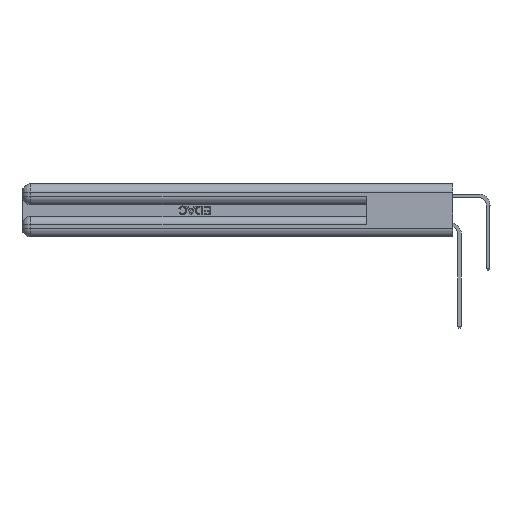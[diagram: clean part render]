
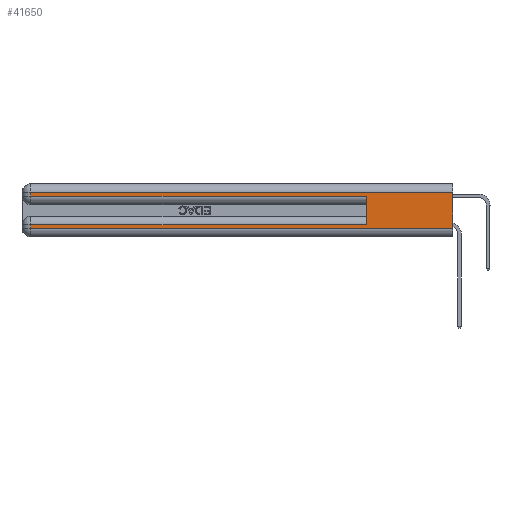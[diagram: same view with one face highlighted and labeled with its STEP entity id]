
A CAD part, left-side view. The second image highlights one B-rep face of the part: STEP entity #41650.
In plain terms, the highlighted planar face has unit normal (-1, 0, 0).
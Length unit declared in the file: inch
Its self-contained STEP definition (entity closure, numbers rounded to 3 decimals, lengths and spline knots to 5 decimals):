
#1185 = CARTESIAN_POINT ( 'NONE',  ( 0., 0.6, 0.145 ) ) ;
#3283 = DIRECTION ( 'NONE',  ( 0., 0., -1. ) ) ;
#3672 = FACE_OUTER_BOUND ( 'NONE', #38801, .T. ) ;
#4326 = CARTESIAN_POINT ( 'NONE',  ( 0., 0., 0.37 ) ) ;
#4602 = DIRECTION ( 'NONE',  ( 0., 0., 1. ) ) ;
#6406 = CARTESIAN_POINT ( 'NONE',  ( 0., 0., 0.31 ) ) ;
#7680 = DIRECTION ( 'NONE',  ( 0., 0., -1. ) ) ;
#8175 = CARTESIAN_POINT ( 'NONE',  ( 0., 2.94, 0.06 ) ) ;
#8320 = EDGE_CURVE ( 'NONE', #40786, #16125, #26603, .T. ) ;
#8511 = VECTOR ( 'NONE', #43599, 39.37008 ) ;
#9150 = AXIS2_PLACEMENT_3D ( 'NONE', #4326, #27938, #7680 ) ;
#9380 = LINE ( 'NONE', #43692, #34223 ) ;
#9932 = CARTESIAN_POINT ( 'NONE',  ( 0., 0., 0.37 ) ) ;
#10296 = VECTOR ( 'NONE', #4602, 39.37008 ) ;
#10394 = CARTESIAN_POINT ( 'NONE',  ( 0., 0., 0.06 ) ) ;
#12262 = ORIENTED_EDGE ( 'NONE', *, *, #25979, .T. ) ;
#12401 = EDGE_CURVE ( 'NONE', #31101, #41060, #9380, .T. ) ;
#14241 = CARTESIAN_POINT ( 'NONE',  ( 0., 0., 0.085 ) ) ;
#14332 = PLANE ( 'NONE',  #9150 ) ;
#14543 = EDGE_CURVE ( 'NONE', #30212, #38504, #37259, .T. ) ;
#16125 = VERTEX_POINT ( 'NONE', #10394 ) ;
#16313 = EDGE_CURVE ( 'NONE', #41060, #16125, #33415, .T. ) ;
#16316 = VECTOR ( 'NONE', #35027, 39.37008 ) ;
#17707 = CARTESIAN_POINT ( 'NONE',  ( 0., 2.94, 0.085 ) ) ;
#18814 = ORIENTED_EDGE ( 'NONE', *, *, #40423, .T. ) ;
#18842 = DIRECTION ( 'NONE',  ( 0., 0., -1. ) ) ;
#20080 = DIRECTION ( 'NONE',  ( 0., 0., -1. ) ) ;
#20556 = VERTEX_POINT ( 'NONE', #24181 ) ;
#20683 = ORIENTED_EDGE ( 'NONE', *, *, #39504, .T. ) ;
#23068 = LINE ( 'NONE', #39111, #31013 ) ;
#23663 = CARTESIAN_POINT ( 'NONE',  ( 0., 0.6, 0.285 ) ) ;
#24181 = CARTESIAN_POINT ( 'NONE',  ( 0., 2.94, 0.285 ) ) ;
#24692 = ORIENTED_EDGE ( 'NONE', *, *, #16313, .T. ) ;
#25609 = CARTESIAN_POINT ( 'NONE',  ( 0., 0.6, 0.085 ) ) ;
#25979 = EDGE_CURVE ( 'NONE', #20556, #38504, #36470, .T. ) ;
#26359 = CARTESIAN_POINT ( 'NONE',  ( 0., 2.94, 0.31 ) ) ;
#26603 = LINE ( 'NONE', #9932, #34559 ) ;
#26878 = ORIENTED_EDGE ( 'NONE', *, *, #14543, .F. ) ;
#27938 = DIRECTION ( 'NONE',  ( 1., 0., 0. ) ) ;
#28336 = VERTEX_POINT ( 'NONE', #26359 ) ;
#28425 = ORIENTED_EDGE ( 'NONE', *, *, #12401, .T. ) ;
#29692 = ORIENTED_EDGE ( 'NONE', *, *, #40972, .T. ) ;
#29718 = CARTESIAN_POINT ( 'NONE',  ( 0., 0., 0.31 ) ) ;
#30212 = VERTEX_POINT ( 'NONE', #25609 ) ;
#31013 = VECTOR ( 'NONE', #18842, 39.37008 ) ;
#31101 = VERTEX_POINT ( 'NONE', #17707 ) ;
#31509 = CARTESIAN_POINT ( 'NONE',  ( 0., 0., 0.06 ) ) ;
#31625 = CARTESIAN_POINT ( 'NONE',  ( 0., 0., 0.285 ) ) ;
#32363 = VECTOR ( 'NONE', #34915, 39.37008 ) ;
#33415 = LINE ( 'NONE', #31509, #32363 ) ;
#34223 = VECTOR ( 'NONE', #3283, 39.37008 ) ;
#34559 = VECTOR ( 'NONE', #20080, 39.37008 ) ;
#34915 = DIRECTION ( 'NONE',  ( 0., -1., 0. ) ) ;
#35027 = DIRECTION ( 'NONE',  ( 0., -1., 0. ) ) ;
#35501 = LINE ( 'NONE', #6406, #8511 ) ;
#36470 = LINE ( 'NONE', #31625, #16316 ) ;
#37259 = LINE ( 'NONE', #1185, #10296 ) ;
#38030 = DIRECTION ( 'NONE',  ( 0., 1., 0. ) ) ;
#38504 = VERTEX_POINT ( 'NONE', #23663 ) ;
#38801 = EDGE_LOOP ( 'NONE', ( #42766, #18814, #20683, #12262, #26878, #29692, #28425, #24692 ) ) ;
#39111 = CARTESIAN_POINT ( 'NONE',  ( 0., 2.94, 0.37 ) ) ;
#39504 = EDGE_CURVE ( 'NONE', #28336, #20556, #23068, .T. ) ;
#40175 = LINE ( 'NONE', #14241, #41220 ) ;
#40423 = EDGE_CURVE ( 'NONE', #40786, #28336, #35501, .T. ) ;
#40786 = VERTEX_POINT ( 'NONE', #29718 ) ;
#40972 = EDGE_CURVE ( 'NONE', #30212, #31101, #40175, .T. ) ;
#41060 = VERTEX_POINT ( 'NONE', #8175 ) ;
#41220 = VECTOR ( 'NONE', #38030, 39.37008 ) ;
#41650 = ADVANCED_FACE ( 'NONE', ( #3672 ), #14332, .F. ) ;
#42766 = ORIENTED_EDGE ( 'NONE', *, *, #8320, .F. ) ;
#43599 = DIRECTION ( 'NONE',  ( 0., 1., 0. ) ) ;
#43692 = CARTESIAN_POINT ( 'NONE',  ( 0., 2.94, 0.37 ) ) ;
